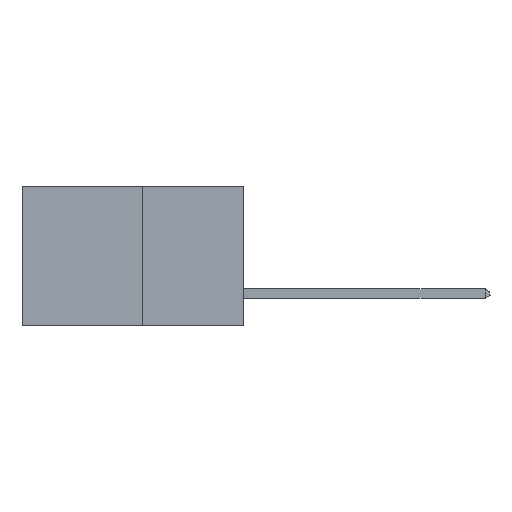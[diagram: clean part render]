
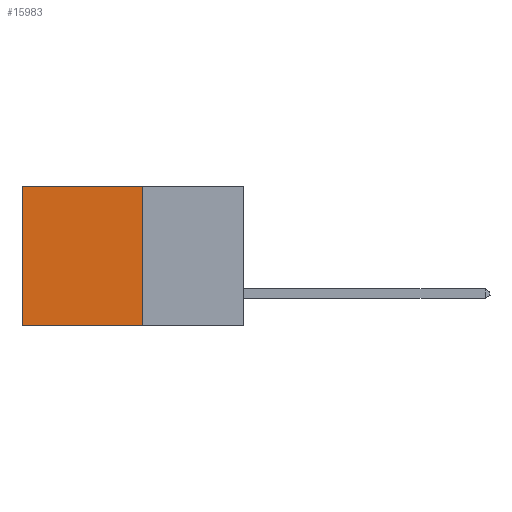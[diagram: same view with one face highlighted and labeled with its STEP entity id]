
A CAD part, left-side view. The second image highlights one B-rep face of the part: STEP entity #15983.
In plain terms, the highlighted planar face has unit normal (-1, 0, 0).
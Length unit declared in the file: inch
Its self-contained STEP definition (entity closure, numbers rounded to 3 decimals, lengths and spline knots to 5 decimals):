
#175 = DIRECTION ( 'NONE',  ( 0., 0., -1. ) ) ;
#343 = CARTESIAN_POINT ( 'NONE',  ( 0.277, 0.27, -0.37 ) ) ;
#676 = EDGE_CURVE ( 'NONE', #1413, #23208, #5463, .T. ) ;
#1413 = VERTEX_POINT ( 'NONE', #4400 ) ;
#1505 = PLANE ( 'NONE',  #20948 ) ;
#1640 = EDGE_CURVE ( 'NONE', #7394, #23208, #8319, .T. ) ;
#2146 = EDGE_CURVE ( 'NONE', #4852, #1413, #10949, .T. ) ;
#4400 = CARTESIAN_POINT ( 'NONE',  ( 0.277, 0.59, 0. ) ) ;
#4852 = VERTEX_POINT ( 'NONE', #17303 ) ;
#5133 = ORIENTED_EDGE ( 'NONE', *, *, #6368, .F. ) ;
#5220 = DIRECTION ( 'NONE',  ( 0., 0., -1. ) ) ;
#5382 = VECTOR ( 'NONE', #175, 39.37008 ) ;
#5463 = LINE ( 'NONE', #12125, #14764 ) ;
#6368 = EDGE_CURVE ( 'NONE', #4852, #7394, #20133, .T. ) ;
#7394 = VERTEX_POINT ( 'NONE', #22366 ) ;
#8319 = LINE ( 'NONE', #12060, #13889 ) ;
#8392 = ORIENTED_EDGE ( 'NONE', *, *, #676, .T. ) ;
#10949 = LINE ( 'NONE', #11817, #15864 ) ;
#11785 = DIRECTION ( 'NONE',  ( 0., 1., 0. ) ) ;
#11817 = CARTESIAN_POINT ( 'NONE',  ( 0.277, 0.27, 0. ) ) ;
#11870 = DIRECTION ( 'NONE',  ( 0., 1., 0. ) ) ;
#12044 = DIRECTION ( 'NONE',  ( 0., 0., -1. ) ) ;
#12060 = CARTESIAN_POINT ( 'NONE',  ( 0.277, 0.27, -0.37 ) ) ;
#12125 = CARTESIAN_POINT ( 'NONE',  ( 0.277, 0.59, -0.37 ) ) ;
#13670 = FACE_OUTER_BOUND ( 'NONE', #22790, .T. ) ;
#13889 = VECTOR ( 'NONE', #11870, 39.37008 ) ;
#14476 = CARTESIAN_POINT ( 'NONE',  ( 0.277, 0.27, -0.37 ) ) ;
#14764 = VECTOR ( 'NONE', #12044, 39.37008 ) ;
#14842 = CARTESIAN_POINT ( 'NONE',  ( 0.277, 0.59, -0.37 ) ) ;
#15864 = VECTOR ( 'NONE', #11785, 39.37008 ) ;
#15983 = ADVANCED_FACE ( 'NONE', ( #13670 ), #1505, .F. ) ;
#16294 = DIRECTION ( 'NONE',  ( 1., 0., 0. ) ) ;
#17303 = CARTESIAN_POINT ( 'NONE',  ( 0.277, 0.27, 0. ) ) ;
#17789 = ORIENTED_EDGE ( 'NONE', *, *, #2146, .T. ) ;
#20123 = ORIENTED_EDGE ( 'NONE', *, *, #1640, .F. ) ;
#20133 = LINE ( 'NONE', #343, #5382 ) ;
#20948 = AXIS2_PLACEMENT_3D ( 'NONE', #14476, #16294, #5220 ) ;
#22366 = CARTESIAN_POINT ( 'NONE',  ( 0.277, 0.27, -0.37 ) ) ;
#22790 = EDGE_LOOP ( 'NONE', ( #8392, #20123, #5133, #17789 ) ) ;
#23208 = VERTEX_POINT ( 'NONE', #14842 ) ;
